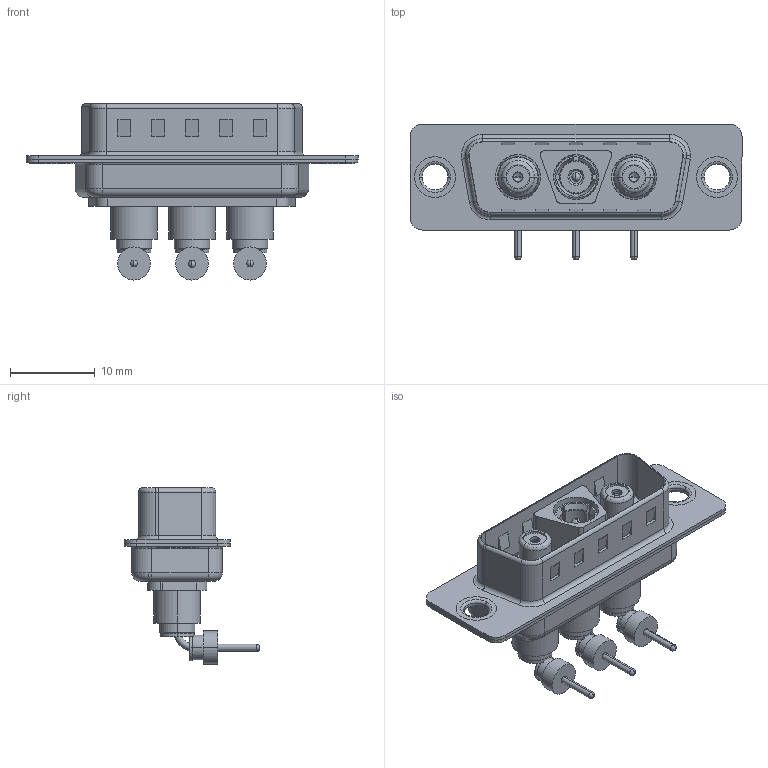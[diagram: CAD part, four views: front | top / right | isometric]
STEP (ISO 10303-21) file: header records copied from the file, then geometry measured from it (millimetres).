
FILE_DESCRIPTION (( 'STEP AP203' ), '1' );
FILE_NAME ('629-3WK3640-7N1.STEP', '2022-05-05T14:06:40', ( '' ), ( '' ), 'SwSTEP 2.0', 'SolidWorks 2020', '' );
FILE_SCHEMA (( 'CONFIG_CONTROL_DESIGN' ));
Length unit declared in the file: millimetre
Products named in the file (17): 629Combo Thru Hole Rivet; Insulator Socket; Co-Ax Plug Assy_RA; 629-3WK3640-7N1; Co-Ax Jack Assy_RA; Socket_RA; Insulator Socket 2; Insulator Pin_Straight PC Tail; Co-Ax Plug_RA PC Tail; 629Combo Shell Rear_15 Contacts; 629Combo Shell Front_15 Contacts; Pin_RA; Locking Collar; 629Combo Housing_3WK3; Co-Ax Jack_RA PC Tail; Insulator RA Pin
Assembly tree (25 placements, depth 3):
  629-3WK3640-7N1
    629Combo Housing_3WK3
    629Combo Shell Rear_15 Contacts
    629Combo Shell Front_15 Contacts
    629Combo Thru Hole Rivet  x2
    Co-Ax Plug Assy_RA
      Co-Ax Plug_RA PC Tail
      Insulator Pin_Straight PC Tail
      Pin_RA
      Locking Collar
      Insulator RA Pin
    Co-Ax Jack Assy_RA
      Co-Ax Jack_RA PC Tail
      Insulator Socket
      Insulator Socket 2
      Locking Collar
      Socket_RA
      Insulator RA Pin
    Co-Ax Jack Assy_RA
      Co-Ax Jack_RA PC Tail
      Insulator Socket
      Insulator Socket 2
      Locking Collar
      Socket_RA
      Insulator RA Pin
Bounding box: 39.2 x 16 x 20.79 mm (x, y, z)
Volume: 2197.4 mm3; surface area: 6480.3 mm2
Topology: 22 solids, 22 shells, 691 faces, 1632 edges, 1024 vertices
Faces by surface type: cylinder 303, plane 256, torus 76, cone 45, sphere 8, bspline 3
Entity records: 18012 total; most frequent: DIRECTION 2967, CARTESIAN_POINT 2897, ORIENTED_EDGE 2568, EDGE_CURVE 1284, AXIS2_PLACEMENT_3D 1159, VERTEX_POINT 812, LINE 649, VECTOR 649
